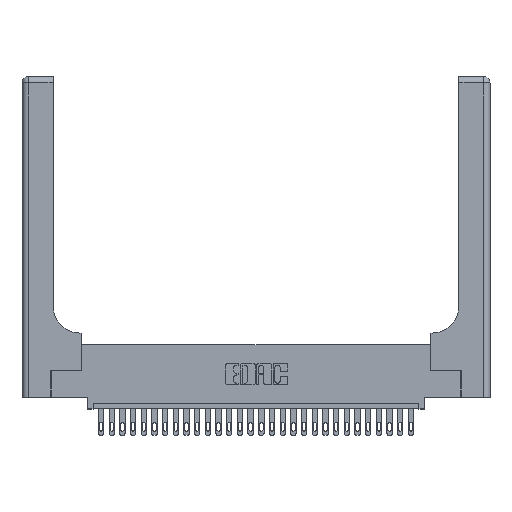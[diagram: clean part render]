
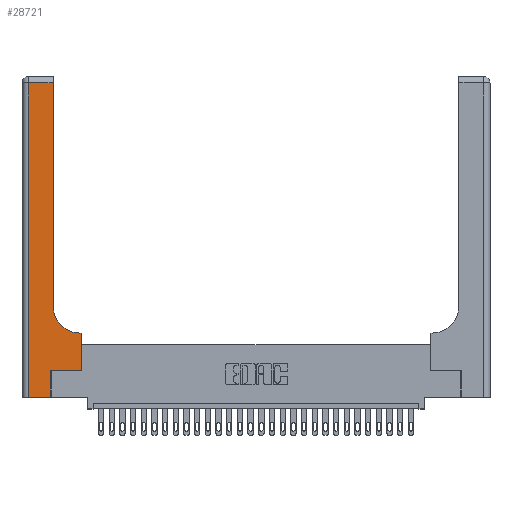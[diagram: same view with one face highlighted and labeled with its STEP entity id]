
A CAD part, top view. The second image highlights one B-rep face of the part: STEP entity #28721.
In plain terms, the highlighted planar face has unit normal (0, 0, 1).
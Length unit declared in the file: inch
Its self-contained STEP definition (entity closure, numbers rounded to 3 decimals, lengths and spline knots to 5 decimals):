
#2178 = EDGE_CURVE ( 'NONE', #4093, #3274, #17996, .T. ) ;
#2258 = CARTESIAN_POINT ( 'NONE',  ( 0.5415, 0.85, 0.37 ) ) ;
#3212 = EDGE_CURVE ( 'NONE', #13603, #4093, #14731, .T. ) ;
#3274 = VERTEX_POINT ( 'NONE', #24113 ) ;
#3428 = LINE ( 'NONE', #25964, #14761 ) ;
#3486 = LINE ( 'NONE', #20128, #13760 ) ;
#3576 = ORIENTED_EDGE ( 'NONE', *, *, #25178, .T. ) ;
#3764 = EDGE_CURVE ( 'NONE', #9833, #13603, #7420, .T. ) ;
#4078 = LINE ( 'NONE', #21531, #27558 ) ;
#4093 = VERTEX_POINT ( 'NONE', #24931 ) ;
#4600 = DIRECTION ( 'NONE',  ( -1., 0., 0. ) ) ;
#5617 = CARTESIAN_POINT ( 'NONE',  ( 0.5585, 0.6, 0.37 ) ) ;
#6072 = FACE_OUTER_BOUND ( 'NONE', #13969, .T. ) ;
#6117 = CARTESIAN_POINT ( 'NONE',  ( 0.5585, 0.25, 0.37 ) ) ;
#7420 = CIRCLE ( 'NONE', #14458, 0.25 ) ;
#7953 = CARTESIAN_POINT ( 'NONE',  ( 0.269, 0., 0.37 ) ) ;
#8371 = DIRECTION ( 'NONE',  ( 0., 0., -1. ) ) ;
#8428 = EDGE_CURVE ( 'NONE', #12309, #25444, #26053, .T. ) ;
#9833 = VERTEX_POINT ( 'NONE', #26458 ) ;
#11072 = CARTESIAN_POINT ( 'NONE',  ( 0.06, 0., 0.37 ) ) ;
#11459 = EDGE_CURVE ( 'NONE', #16381, #12309, #4078, .T. ) ;
#11763 = EDGE_CURVE ( 'NONE', #22678, #20739, #29338, .T. ) ;
#12309 = VERTEX_POINT ( 'NONE', #7953 ) ;
#12703 = DIRECTION ( 'NONE',  ( -1., 0., 0. ) ) ;
#12892 = DIRECTION ( 'NONE',  ( -1., 0., 0. ) ) ;
#13493 = ORIENTED_EDGE ( 'NONE', *, *, #3212, .T. ) ;
#13603 = VERTEX_POINT ( 'NONE', #26505 ) ;
#13760 = VECTOR ( 'NONE', #4600, 39.37008 ) ;
#13815 = DIRECTION ( 'NONE',  ( 1., 0., 0. ) ) ;
#13969 = EDGE_LOOP ( 'NONE', ( #13493, #29354, #17637, #27201, #25069, #3576, #26040, #24281, #19216 ) ) ;
#14458 = AXIS2_PLACEMENT_3D ( 'NONE', #2258, #22716, #13815 ) ;
#14731 = LINE ( 'NONE', #24906, #15076 ) ;
#14761 = VECTOR ( 'NONE', #19276, 39.37008 ) ;
#15076 = VECTOR ( 'NONE', #17586, 39.37008 ) ;
#15488 = LINE ( 'NONE', #25245, #18000 ) ;
#15523 = VECTOR ( 'NONE', #12892, 39.37008 ) ;
#16381 = VERTEX_POINT ( 'NONE', #11072 ) ;
#17542 = VECTOR ( 'NONE', #19368, 39.37008 ) ;
#17586 = DIRECTION ( 'NONE',  ( 0., 1., 0. ) ) ;
#17637 = ORIENTED_EDGE ( 'NONE', *, *, #25417, .T. ) ;
#17996 = LINE ( 'NONE', #24403, #15523 ) ;
#18000 = VECTOR ( 'NONE', #20532, 39.37008 ) ;
#19216 = ORIENTED_EDGE ( 'NONE', *, *, #3764, .T. ) ;
#19276 = DIRECTION ( 'NONE',  ( 1., 0., 0. ) ) ;
#19368 = DIRECTION ( 'NONE',  ( 0., 1., 0. ) ) ;
#19502 = CARTESIAN_POINT ( 'NONE',  ( 0., 3., 0.37 ) ) ;
#20128 = CARTESIAN_POINT ( 'NONE',  ( 0.2915, 0.6, 0.37 ) ) ;
#20532 = DIRECTION ( 'NONE',  ( 0., -1., 0. ) ) ;
#20623 = CARTESIAN_POINT ( 'NONE',  ( 0.269, 0.25, 0.37 ) ) ;
#20739 = VERTEX_POINT ( 'NONE', #5617 ) ;
#20996 = EDGE_CURVE ( 'NONE', #20739, #9833, #3486, .T. ) ;
#21215 = DIRECTION ( 'NONE',  ( 0., 1., 0. ) ) ;
#21531 = CARTESIAN_POINT ( 'NONE',  ( 0., 0., 0.37 ) ) ;
#21734 = DIRECTION ( 'NONE',  ( 1., 0., 0. ) ) ;
#22090 = PLANE ( 'NONE',  #27707 ) ;
#22678 = VERTEX_POINT ( 'NONE', #6117 ) ;
#22716 = DIRECTION ( 'NONE',  ( 0., 0., -1. ) ) ;
#23921 = VECTOR ( 'NONE', #21215, 39.37008 ) ;
#24113 = CARTESIAN_POINT ( 'NONE',  ( 0.06, 2.94, 0.37 ) ) ;
#24281 = ORIENTED_EDGE ( 'NONE', *, *, #20996, .T. ) ;
#24403 = CARTESIAN_POINT ( 'NONE',  ( 0., 2.94, 0.37 ) ) ;
#24906 = CARTESIAN_POINT ( 'NONE',  ( 0.2915, 3., 0.37 ) ) ;
#24931 = CARTESIAN_POINT ( 'NONE',  ( 0.2915, 2.94, 0.37 ) ) ;
#25069 = ORIENTED_EDGE ( 'NONE', *, *, #8428, .T. ) ;
#25178 = EDGE_CURVE ( 'NONE', #25444, #22678, #3428, .T. ) ;
#25245 = CARTESIAN_POINT ( 'NONE',  ( 0.06, 3., 0.37 ) ) ;
#25417 = EDGE_CURVE ( 'NONE', #3274, #16381, #15488, .T. ) ;
#25444 = VERTEX_POINT ( 'NONE', #20623 ) ;
#25964 = CARTESIAN_POINT ( 'NONE',  ( 0.269, 0.25, 0.37 ) ) ;
#26040 = ORIENTED_EDGE ( 'NONE', *, *, #11763, .T. ) ;
#26053 = LINE ( 'NONE', #28200, #23921 ) ;
#26458 = CARTESIAN_POINT ( 'NONE',  ( 0.5415, 0.6, 0.37 ) ) ;
#26505 = CARTESIAN_POINT ( 'NONE',  ( 0.2915, 0.85, 0.37 ) ) ;
#27201 = ORIENTED_EDGE ( 'NONE', *, *, #11459, .T. ) ;
#27558 = VECTOR ( 'NONE', #21734, 39.37008 ) ;
#27707 = AXIS2_PLACEMENT_3D ( 'NONE', #19502, #8371, #12703 ) ;
#28200 = CARTESIAN_POINT ( 'NONE',  ( 0.269, 0., 0.37 ) ) ;
#28535 = CARTESIAN_POINT ( 'NONE',  ( 0.5585, 0.25, 0.37 ) ) ;
#28721 = ADVANCED_FACE ( 'NONE', ( #6072 ), #22090, .F. ) ;
#29338 = LINE ( 'NONE', #28535, #17542 ) ;
#29354 = ORIENTED_EDGE ( 'NONE', *, *, #2178, .T. ) ;
